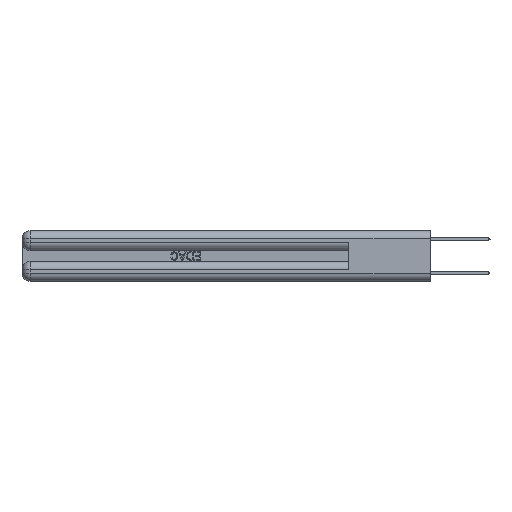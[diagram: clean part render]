
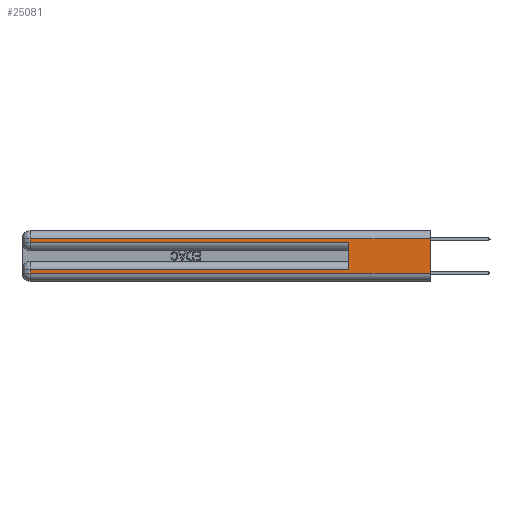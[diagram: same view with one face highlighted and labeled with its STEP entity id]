
A CAD part, left-side view. The second image highlights one B-rep face of the part: STEP entity #25081.
In plain terms, the highlighted planar face has unit normal (-1, 0, 0).
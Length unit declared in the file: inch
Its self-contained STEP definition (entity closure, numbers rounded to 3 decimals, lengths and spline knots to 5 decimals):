
#1069 = ORIENTED_EDGE ( 'NONE', *, *, #29369, .T. ) ;
#1183 = VERTEX_POINT ( 'NONE', #5811 ) ;
#1847 = ORIENTED_EDGE ( 'NONE', *, *, #3849, .F. ) ;
#1925 = EDGE_CURVE ( 'NONE', #11972, #13891, #14869, .T. ) ;
#1942 = CARTESIAN_POINT ( 'NONE',  ( 0., 0., 0.31 ) ) ;
#2610 = VERTEX_POINT ( 'NONE', #26491 ) ;
#3397 = CARTESIAN_POINT ( 'NONE',  ( 0., 2.94, 0.37 ) ) ;
#3849 = EDGE_CURVE ( 'NONE', #2610, #14086, #11463, .T. ) ;
#4173 = VECTOR ( 'NONE', #25642, 39.37008 ) ;
#5798 = PLANE ( 'NONE',  #13654 ) ;
#5811 = CARTESIAN_POINT ( 'NONE',  ( 0., 2.94, 0.31 ) ) ;
#6995 = EDGE_CURVE ( 'NONE', #13891, #16024, #13220, .T. ) ;
#8085 = DIRECTION ( 'NONE',  ( 1., 0., 0. ) ) ;
#8105 = VECTOR ( 'NONE', #32285, 39.37008 ) ;
#8380 = DIRECTION ( 'NONE',  ( 0., 0., -1. ) ) ;
#9446 = CARTESIAN_POINT ( 'NONE',  ( 0., 0., 0.06 ) ) ;
#10606 = DIRECTION ( 'NONE',  ( 0., 0., 1. ) ) ;
#10891 = LINE ( 'NONE', #30640, #4173 ) ;
#11463 = LINE ( 'NONE', #13209, #27601 ) ;
#11692 = ORIENTED_EDGE ( 'NONE', *, *, #16471, .T. ) ;
#11963 = VECTOR ( 'NONE', #24575, 39.37008 ) ;
#11972 = VERTEX_POINT ( 'NONE', #24962 ) ;
#12453 = CARTESIAN_POINT ( 'NONE',  ( 0., 2.94, 0.06 ) ) ;
#13209 = CARTESIAN_POINT ( 'NONE',  ( 0., 0.6, 0.145 ) ) ;
#13220 = LINE ( 'NONE', #9446, #8105 ) ;
#13466 = ORIENTED_EDGE ( 'NONE', *, *, #6995, .T. ) ;
#13561 = LINE ( 'NONE', #1942, #26193 ) ;
#13654 = AXIS2_PLACEMENT_3D ( 'NONE', #20619, #8085, #18110 ) ;
#13891 = VERTEX_POINT ( 'NONE', #12453 ) ;
#14086 = VERTEX_POINT ( 'NONE', #23666 ) ;
#14869 = LINE ( 'NONE', #17961, #19610 ) ;
#15096 = EDGE_CURVE ( 'NONE', #18352, #16024, #20605, .T. ) ;
#16024 = VERTEX_POINT ( 'NONE', #28409 ) ;
#16471 = EDGE_CURVE ( 'NONE', #2610, #11972, #32230, .T. ) ;
#16657 = DIRECTION ( 'NONE',  ( 0., 1., 0. ) ) ;
#16683 = ORIENTED_EDGE ( 'NONE', *, *, #17537, .T. ) ;
#17276 = VERTEX_POINT ( 'NONE', #29649 ) ;
#17537 = EDGE_CURVE ( 'NONE', #17276, #14086, #10891, .T. ) ;
#17925 = EDGE_CURVE ( 'NONE', #18352, #1183, #13561, .T. ) ;
#17961 = CARTESIAN_POINT ( 'NONE',  ( 0., 2.94, 0.37 ) ) ;
#18110 = DIRECTION ( 'NONE',  ( 0., 0., -1. ) ) ;
#18306 = LINE ( 'NONE', #3397, #26921 ) ;
#18352 = VERTEX_POINT ( 'NONE', #29204 ) ;
#19610 = VECTOR ( 'NONE', #8380, 39.37008 ) ;
#20230 = ORIENTED_EDGE ( 'NONE', *, *, #17925, .T. ) ;
#20605 = LINE ( 'NONE', #22057, #11963 ) ;
#20619 = CARTESIAN_POINT ( 'NONE',  ( 0., 0., 0.37 ) ) ;
#20807 = FACE_OUTER_BOUND ( 'NONE', #24209, .T. ) ;
#22057 = CARTESIAN_POINT ( 'NONE',  ( 0., 0., 0.37 ) ) ;
#23597 = DIRECTION ( 'NONE',  ( 0., 1., 0. ) ) ;
#23666 = CARTESIAN_POINT ( 'NONE',  ( 0., 0.6, 0.285 ) ) ;
#24209 = EDGE_LOOP ( 'NONE', ( #27751, #20230, #1069, #16683, #1847, #11692, #25745, #13466 ) ) ;
#24575 = DIRECTION ( 'NONE',  ( 0., 0., -1. ) ) ;
#24962 = CARTESIAN_POINT ( 'NONE',  ( 0., 2.94, 0.085 ) ) ;
#25081 = ADVANCED_FACE ( 'NONE', ( #20807 ), #5798, .F. ) ;
#25642 = DIRECTION ( 'NONE',  ( 0., -1., 0. ) ) ;
#25745 = ORIENTED_EDGE ( 'NONE', *, *, #1925, .T. ) ;
#26193 = VECTOR ( 'NONE', #16657, 39.37008 ) ;
#26288 = VECTOR ( 'NONE', #23597, 39.37008 ) ;
#26491 = CARTESIAN_POINT ( 'NONE',  ( 0., 0.6, 0.085 ) ) ;
#26921 = VECTOR ( 'NONE', #31164, 39.37008 ) ;
#27601 = VECTOR ( 'NONE', #10606, 39.37008 ) ;
#27751 = ORIENTED_EDGE ( 'NONE', *, *, #15096, .F. ) ;
#28409 = CARTESIAN_POINT ( 'NONE',  ( 0., 0., 0.06 ) ) ;
#29204 = CARTESIAN_POINT ( 'NONE',  ( 0., 0., 0.31 ) ) ;
#29369 = EDGE_CURVE ( 'NONE', #1183, #17276, #18306, .T. ) ;
#29649 = CARTESIAN_POINT ( 'NONE',  ( 0., 2.94, 0.285 ) ) ;
#30640 = CARTESIAN_POINT ( 'NONE',  ( 0., 0., 0.285 ) ) ;
#31164 = DIRECTION ( 'NONE',  ( 0., 0., -1. ) ) ;
#31252 = CARTESIAN_POINT ( 'NONE',  ( 0., 0., 0.085 ) ) ;
#32230 = LINE ( 'NONE', #31252, #26288 ) ;
#32285 = DIRECTION ( 'NONE',  ( 0., -1., 0. ) ) ;
